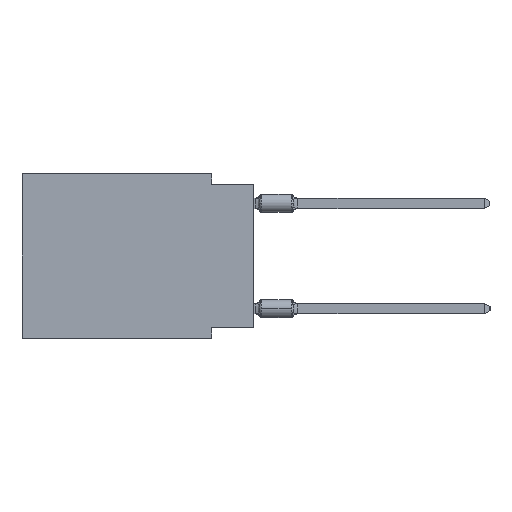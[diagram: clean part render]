
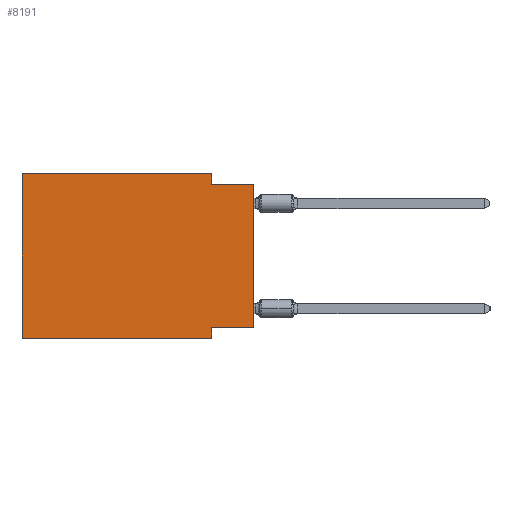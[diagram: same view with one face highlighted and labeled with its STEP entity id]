
A CAD part, left-side view. The second image highlights one B-rep face of the part: STEP entity #8191.
In plain terms, the highlighted planar face has unit normal (-1, 0, 0).
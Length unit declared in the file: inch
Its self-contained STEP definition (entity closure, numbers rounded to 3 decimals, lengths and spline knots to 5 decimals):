
#112 = EDGE_CURVE ( 'NONE', #15490, #31286, #20457, .T. ) ;
#689 = DIRECTION ( 'NONE',  ( 0., -1., 0. ) ) ;
#1529 = LINE ( 'NONE', #24240, #23349 ) ;
#2369 = EDGE_CURVE ( 'NONE', #32921, #5438, #35449, .T. ) ;
#2965 = ORIENTED_EDGE ( 'NONE', *, *, #11823, .F. ) ;
#3165 = DIRECTION ( 'NONE',  ( 0., 0., -1. ) ) ;
#3335 = DIRECTION ( 'NONE',  ( 1., 0., 0. ) ) ;
#3360 = VERTEX_POINT ( 'NONE', #14278 ) ;
#3428 = EDGE_CURVE ( 'NONE', #13296, #20976, #14047, .T. ) ;
#4524 = EDGE_CURVE ( 'NONE', #13296, #15962, #32007, .T. ) ;
#4719 = CARTESIAN_POINT ( 'NONE',  ( 0., 0., 0. ) ) ;
#5438 = VERTEX_POINT ( 'NONE', #27421 ) ;
#5548 = ORIENTED_EDGE ( 'NONE', *, *, #112, .F. ) ;
#5944 = CARTESIAN_POINT ( 'NONE',  ( 0., 0.1, 0. ) ) ;
#6469 = CARTESIAN_POINT ( 'NONE',  ( 0., 0.55, 0. ) ) ;
#6684 = FACE_OUTER_BOUND ( 'NONE', #32021, .T. ) ;
#8191 = ADVANCED_FACE ( 'NONE', ( #6684 ), #28868, .F. ) ;
#8283 = DIRECTION ( 'NONE',  ( 0., -1., 0. ) ) ;
#8341 = AXIS2_PLACEMENT_3D ( 'NONE', #18007, #3335, #14685 ) ;
#9172 = LINE ( 'NONE', #14393, #9705 ) ;
#9418 = ORIENTED_EDGE ( 'NONE', *, *, #36652, .F. ) ;
#9628 = VECTOR ( 'NONE', #3165, 39.37008 ) ;
#9705 = VECTOR ( 'NONE', #20529, 39.37008 ) ;
#11689 = CARTESIAN_POINT ( 'NONE',  ( 0., 0.55, 0. ) ) ;
#11823 = EDGE_CURVE ( 'NONE', #32921, #3360, #9172, .T. ) ;
#12016 = ORIENTED_EDGE ( 'NONE', *, *, #2369, .T. ) ;
#12798 = VECTOR ( 'NONE', #18672, 39.37008 ) ;
#13225 = DIRECTION ( 'NONE',  ( 0., -1., 0. ) ) ;
#13296 = VERTEX_POINT ( 'NONE', #30605 ) ;
#13347 = VECTOR ( 'NONE', #17798, 39.37008 ) ;
#13682 = CARTESIAN_POINT ( 'NONE',  ( 0., 0.55, -0.39 ) ) ;
#14018 = CARTESIAN_POINT ( 'NONE',  ( 0., 0., -0.365 ) ) ;
#14047 = LINE ( 'NONE', #13682, #21749 ) ;
#14278 = CARTESIAN_POINT ( 'NONE',  ( 0., 0.1, -0.365 ) ) ;
#14393 = CARTESIAN_POINT ( 'NONE',  ( 0., 0., -0.365 ) ) ;
#14527 = ORIENTED_EDGE ( 'NONE', *, *, #28045, .F. ) ;
#14685 = DIRECTION ( 'NONE',  ( 0., 0., -1. ) ) ;
#15398 = ORIENTED_EDGE ( 'NONE', *, *, #4524, .F. ) ;
#15490 = VERTEX_POINT ( 'NONE', #25182 ) ;
#15962 = VERTEX_POINT ( 'NONE', #11689 ) ;
#17438 = ORIENTED_EDGE ( 'NONE', *, *, #3428, .T. ) ;
#17798 = DIRECTION ( 'NONE',  ( 0., 0., 1. ) ) ;
#18007 = CARTESIAN_POINT ( 'NONE',  ( 0., 0.55, 0. ) ) ;
#18394 = VECTOR ( 'NONE', #24931, 39.37008 ) ;
#18672 = DIRECTION ( 'NONE',  ( 0., 0., 1. ) ) ;
#19865 = LINE ( 'NONE', #28274, #36114 ) ;
#20181 = ORIENTED_EDGE ( 'NONE', *, *, #30756, .F. ) ;
#20373 = CARTESIAN_POINT ( 'NONE',  ( 0., 0.1, -0.025 ) ) ;
#20457 = LINE ( 'NONE', #5944, #9628 ) ;
#20529 = DIRECTION ( 'NONE',  ( 0., 1., 0. ) ) ;
#20976 = VERTEX_POINT ( 'NONE', #32351 ) ;
#21749 = VECTOR ( 'NONE', #8283, 39.37008 ) ;
#23349 = VECTOR ( 'NONE', #13225, 39.37008 ) ;
#24240 = CARTESIAN_POINT ( 'NONE',  ( 0., 0.55, 0. ) ) ;
#24931 = DIRECTION ( 'NONE',  ( 0., 0., -1. ) ) ;
#25121 = CARTESIAN_POINT ( 'NONE',  ( 0., 0.1, -0.39 ) ) ;
#25182 = CARTESIAN_POINT ( 'NONE',  ( 0., 0.1, 0. ) ) ;
#27421 = CARTESIAN_POINT ( 'NONE',  ( 0., 0., -0.025 ) ) ;
#28045 = EDGE_CURVE ( 'NONE', #31286, #5438, #19865, .T. ) ;
#28274 = CARTESIAN_POINT ( 'NONE',  ( 0., 0., -0.025 ) ) ;
#28868 = PLANE ( 'NONE',  #8341 ) ;
#30605 = CARTESIAN_POINT ( 'NONE',  ( 0., 0.55, -0.39 ) ) ;
#30756 = EDGE_CURVE ( 'NONE', #3360, #20976, #34006, .T. ) ;
#31286 = VERTEX_POINT ( 'NONE', #20373 ) ;
#32007 = LINE ( 'NONE', #6469, #13347 ) ;
#32021 = EDGE_LOOP ( 'NONE', ( #12016, #14527, #5548, #9418, #15398, #17438, #20181, #2965 ) ) ;
#32351 = CARTESIAN_POINT ( 'NONE',  ( 0., 0.1, -0.39 ) ) ;
#32921 = VERTEX_POINT ( 'NONE', #14018 ) ;
#34006 = LINE ( 'NONE', #25121, #18394 ) ;
#35449 = LINE ( 'NONE', #4719, #12798 ) ;
#36114 = VECTOR ( 'NONE', #689, 39.37008 ) ;
#36652 = EDGE_CURVE ( 'NONE', #15962, #15490, #1529, .T. ) ;
